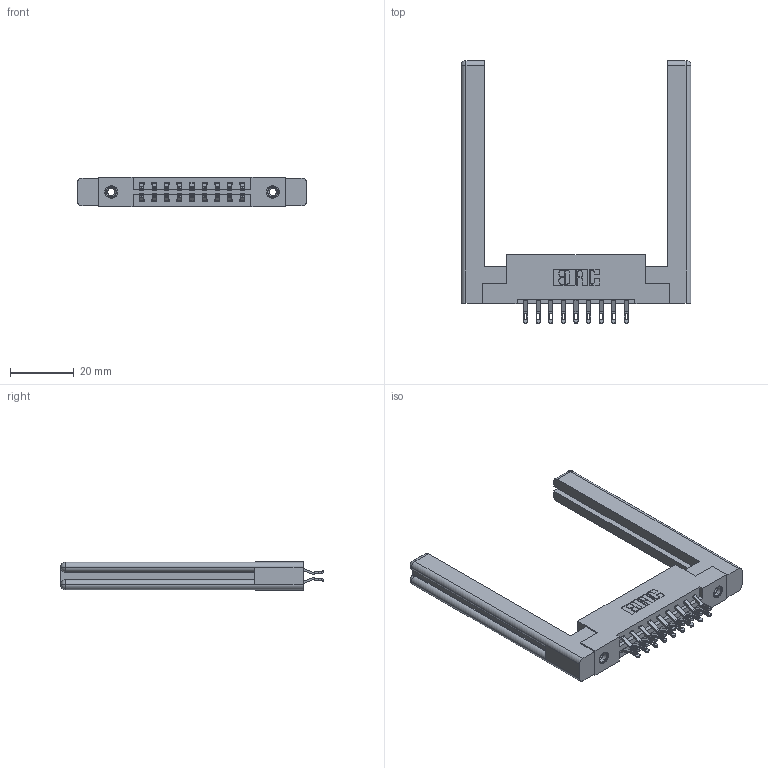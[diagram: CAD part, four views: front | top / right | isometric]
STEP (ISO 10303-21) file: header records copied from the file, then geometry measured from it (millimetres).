
FILE_DESCRIPTION (( 'STEP AP203' ), '1' );
FILE_NAME ('337-018-555-258.STEP', '2019-10-08T13:24:44', ( '' ), ( '' ), 'SwSTEP 2.0', 'SolidWorks 2016', '' );
FILE_SCHEMA (( 'CONFIG_CONTROL_DESIGN' ));
Length unit declared in the file: inch
Products named in the file (5): 345-250-001_345-250-001-102; 337-018-555-258; 345-292-001_555 Tail; 307-220-058; 337 Part_Flush Mounting Lugs - 0.156 Dia-TI
Assembly tree (23 placements, depth 2):
  337-018-555-258
    337 Part_Flush Mounting Lugs - 0.156 Dia-TI
    345-292-001_555 Tail  x18
    345-250-001_345-250-001-102  x2
    307-220-058  x2
Bounding box: 72.29 x 82.56 x 9.4 mm (x, y, z)
Volume: 14373.6 mm3; surface area: 13097.9 mm2
Topology: 23 solids, 23 shells, 1336 faces, 4067 edges, 2698 vertices
Faces by surface type: plane 802, cylinder 510, cone 12, torus 12
Entity records: 14206 total; most frequent: CARTESIAN_POINT 2463, ORIENTED_EDGE 2308, DIRECTION 2142, EDGE_CURVE 1154, VECTOR 958, LINE 958, VERTEX_POINT 762, AXIS2_PLACEMENT_3D 592
